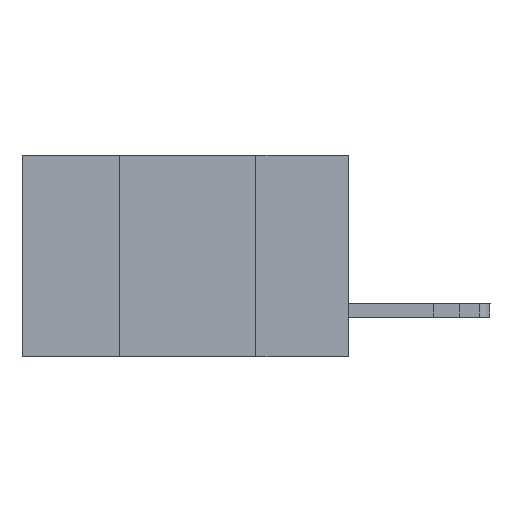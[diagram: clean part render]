
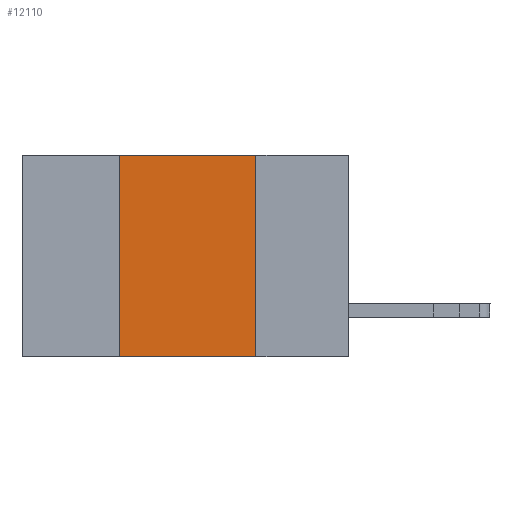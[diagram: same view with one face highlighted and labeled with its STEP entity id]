
A CAD part, left-side view. The second image highlights one B-rep face of the part: STEP entity #12110.
In plain terms, the highlighted planar face has unit normal (-1, 0, 0).
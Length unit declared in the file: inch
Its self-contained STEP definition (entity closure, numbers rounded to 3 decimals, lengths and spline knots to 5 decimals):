
#55 = PLANE ( 'NONE',  #3225 ) ;
#115 = DIRECTION ( 'NONE',  ( 1., 0., 0. ) ) ;
#747 = EDGE_CURVE ( 'NONE', #10425, #2646, #8436, .T. ) ;
#1267 = DIRECTION ( 'NONE',  ( 0., 0., -1. ) ) ;
#1396 = DIRECTION ( 'NONE',  ( 0., 0., -1. ) ) ;
#1459 = CARTESIAN_POINT ( 'NONE',  ( 0., 0.17, 0. ) ) ;
#2646 = VERTEX_POINT ( 'NONE', #5471 ) ;
#2887 = VECTOR ( 'NONE', #10716, 39.37008 ) ;
#3013 = VECTOR ( 'NONE', #6459, 39.37008 ) ;
#3225 = AXIS2_PLACEMENT_3D ( 'NONE', #8357, #115, #1267 ) ;
#3661 = ORIENTED_EDGE ( 'NONE', *, *, #747, .F. ) ;
#3942 = EDGE_CURVE ( 'NONE', #2646, #9998, #10710, .T. ) ;
#4845 = ORIENTED_EDGE ( 'NONE', *, *, #3942, .F. ) ;
#5471 = CARTESIAN_POINT ( 'NONE',  ( 0., 0.17, 0. ) ) ;
#5902 = ORIENTED_EDGE ( 'NONE', *, *, #6003, .F. ) ;
#6003 = EDGE_CURVE ( 'NONE', #10154, #10425, #10850, .T. ) ;
#6241 = EDGE_CURVE ( 'NONE', #10154, #9998, #10974, .T. ) ;
#6392 = CARTESIAN_POINT ( 'NONE',  ( 0., 0.42, 0. ) ) ;
#6459 = DIRECTION ( 'NONE',  ( 0., -1., 0. ) ) ;
#6829 = CARTESIAN_POINT ( 'NONE',  ( 0., 0.6, -0.37 ) ) ;
#7503 = ORIENTED_EDGE ( 'NONE', *, *, #6241, .T. ) ;
#8058 = DIRECTION ( 'NONE',  ( 0., -1., 0. ) ) ;
#8289 = FACE_OUTER_BOUND ( 'NONE', #12872, .T. ) ;
#8357 = CARTESIAN_POINT ( 'NONE',  ( 0., 0.6, 0. ) ) ;
#8436 = LINE ( 'NONE', #8509, #3013 ) ;
#8509 = CARTESIAN_POINT ( 'NONE',  ( 0., 0.6, 0. ) ) ;
#8713 = VECTOR ( 'NONE', #1396, 39.37008 ) ;
#9625 = VECTOR ( 'NONE', #8058, 39.37008 ) ;
#9998 = VERTEX_POINT ( 'NONE', #11646 ) ;
#10154 = VERTEX_POINT ( 'NONE', #12808 ) ;
#10425 = VERTEX_POINT ( 'NONE', #6392 ) ;
#10710 = LINE ( 'NONE', #1459, #8713 ) ;
#10716 = DIRECTION ( 'NONE',  ( 0., 0., 1. ) ) ;
#10850 = LINE ( 'NONE', #12711, #2887 ) ;
#10974 = LINE ( 'NONE', #6829, #9625 ) ;
#11646 = CARTESIAN_POINT ( 'NONE',  ( 0., 0.17, -0.37 ) ) ;
#12110 = ADVANCED_FACE ( 'NONE', ( #8289 ), #55, .F. ) ;
#12711 = CARTESIAN_POINT ( 'NONE',  ( 0., 0.42, 0. ) ) ;
#12808 = CARTESIAN_POINT ( 'NONE',  ( 0., 0.42, -0.37 ) ) ;
#12872 = EDGE_LOOP ( 'NONE', ( #4845, #3661, #5902, #7503 ) ) ;
